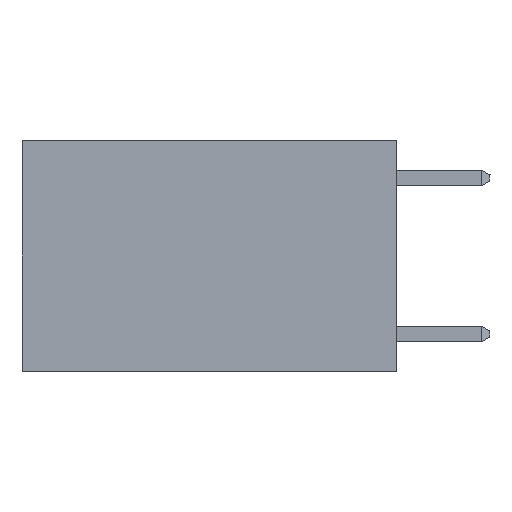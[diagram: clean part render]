
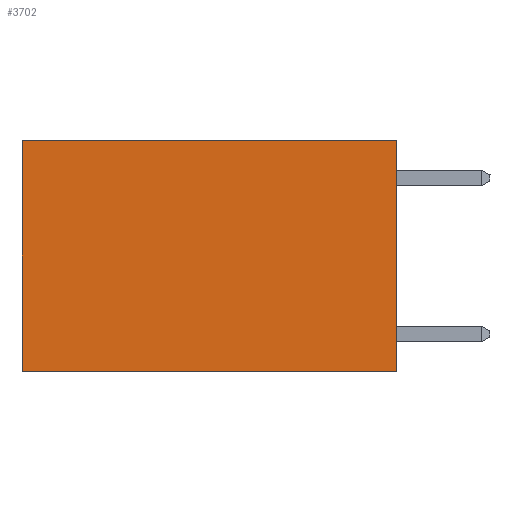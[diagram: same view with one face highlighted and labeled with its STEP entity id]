
A CAD part, left-side view. The second image highlights one B-rep face of the part: STEP entity #3702.
In plain terms, the highlighted planar face has unit normal (-1, 0, 0).
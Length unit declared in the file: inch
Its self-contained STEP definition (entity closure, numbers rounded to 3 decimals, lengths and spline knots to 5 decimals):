
#135 = LINE ( 'NONE', #1300, #13161 ) ;
#185 = VECTOR ( 'NONE', #7022, 39.37008 ) ;
#1300 = CARTESIAN_POINT ( 'NONE',  ( 0.2625, 0., 0. ) ) ;
#1371 = EDGE_CURVE ( 'NONE', #11388, #12809, #14799, .T. ) ;
#1929 = CARTESIAN_POINT ( 'NONE',  ( 0.2625, 0., -0.37 ) ) ;
#2439 = PLANE ( 'NONE',  #6705 ) ;
#3246 = LINE ( 'NONE', #1929, #185 ) ;
#3702 = ADVANCED_FACE ( 'NONE', ( #15201 ), #2439, .F. ) ;
#3917 = DIRECTION ( 'NONE',  ( 0., 0., -1. ) ) ;
#4702 = CARTESIAN_POINT ( 'NONE',  ( 0.2625, 0., 0. ) ) ;
#4779 = ORIENTED_EDGE ( 'NONE', *, *, #1371, .F. ) ;
#4937 = ORIENTED_EDGE ( 'NONE', *, *, #8901, .T. ) ;
#4997 = DIRECTION ( 'NONE',  ( 0., 0., -1. ) ) ;
#5748 = ORIENTED_EDGE ( 'NONE', *, *, #14565, .F. ) ;
#6456 = DIRECTION ( 'NONE',  ( 0., 1., 0. ) ) ;
#6705 = AXIS2_PLACEMENT_3D ( 'NONE', #11232, #12470, #4997 ) ;
#7022 = DIRECTION ( 'NONE',  ( 0., 1., 0. ) ) ;
#7560 = VERTEX_POINT ( 'NONE', #14037 ) ;
#8030 = VERTEX_POINT ( 'NONE', #9937 ) ;
#8901 = EDGE_CURVE ( 'NONE', #7560, #8030, #10491, .T. ) ;
#9570 = EDGE_CURVE ( 'NONE', #11388, #7560, #135, .T. ) ;
#9937 = CARTESIAN_POINT ( 'NONE',  ( 0.2625, 0.6, -0.37 ) ) ;
#10491 = LINE ( 'NONE', #13888, #13741 ) ;
#10962 = CARTESIAN_POINT ( 'NONE',  ( 0.2625, 0., -0.37 ) ) ;
#11232 = CARTESIAN_POINT ( 'NONE',  ( 0.2625, 0., 0. ) ) ;
#11363 = ORIENTED_EDGE ( 'NONE', *, *, #9570, .T. ) ;
#11380 = CARTESIAN_POINT ( 'NONE',  ( 0.2625, 0., 0. ) ) ;
#11388 = VERTEX_POINT ( 'NONE', #4702 ) ;
#12470 = DIRECTION ( 'NONE',  ( 1., 0., 0. ) ) ;
#12630 = DIRECTION ( 'NONE',  ( 0., 0., -1. ) ) ;
#12809 = VERTEX_POINT ( 'NONE', #10962 ) ;
#13161 = VECTOR ( 'NONE', #6456, 39.37008 ) ;
#13741 = VECTOR ( 'NONE', #3917, 39.37008 ) ;
#13888 = CARTESIAN_POINT ( 'NONE',  ( 0.2625, 0.6, 0. ) ) ;
#14037 = CARTESIAN_POINT ( 'NONE',  ( 0.2625, 0.6, 0. ) ) ;
#14415 = VECTOR ( 'NONE', #12630, 39.37008 ) ;
#14565 = EDGE_CURVE ( 'NONE', #12809, #8030, #3246, .T. ) ;
#14570 = EDGE_LOOP ( 'NONE', ( #4937, #5748, #4779, #11363 ) ) ;
#14799 = LINE ( 'NONE', #11380, #14415 ) ;
#15201 = FACE_OUTER_BOUND ( 'NONE', #14570, .T. ) ;
